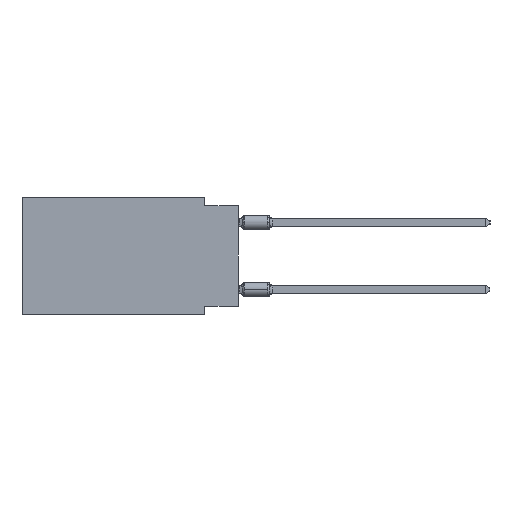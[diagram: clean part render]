
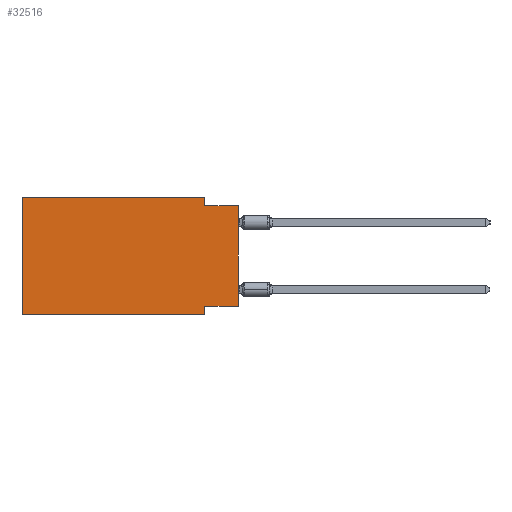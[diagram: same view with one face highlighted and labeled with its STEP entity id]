
A CAD part, left-side view. The second image highlights one B-rep face of the part: STEP entity #32516.
In plain terms, the highlighted planar face has unit normal (-1, 0, 0).
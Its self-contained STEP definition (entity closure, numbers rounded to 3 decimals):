
#209 = LINE ( 'NONE', #14138, #35410 ) ;
#517 = EDGE_CURVE ( 'NONE', #12664, #16205, #19904, .T. ) ;
#721 = EDGE_CURVE ( 'NONE', #12664, #32667, #12485, .T. ) ;
#1262 = CARTESIAN_POINT ( 'NONE',  ( 0., 2.54, -8.255 ) ) ;
#1575 = CARTESIAN_POINT ( 'NONE',  ( 0., 2.54, 0. ) ) ;
#2400 = CARTESIAN_POINT ( 'NONE',  ( 0., 16.383, 0. ) ) ;
#2664 = EDGE_CURVE ( 'NONE', #16205, #27501, #15067, .T. ) ;
#3215 = CARTESIAN_POINT ( 'NONE',  ( 0., 0., -0.635 ) ) ;
#3784 = CARTESIAN_POINT ( 'NONE',  ( 0., 0., -0.635 ) ) ;
#4337 = CARTESIAN_POINT ( 'NONE',  ( 0., 16.383, 0. ) ) ;
#5484 = VECTOR ( 'NONE', #33644, 1000. ) ;
#5692 = ORIENTED_EDGE ( 'NONE', *, *, #2664, .F. ) ;
#7178 = EDGE_CURVE ( 'NONE', #9628, #32667, #209, .T. ) ;
#7376 = DIRECTION ( 'NONE',  ( 1., 0., 0. ) ) ;
#7545 = CARTESIAN_POINT ( 'NONE',  ( 0., 0., -8.255 ) ) ;
#7728 = LINE ( 'NONE', #7545, #30053 ) ;
#8511 = EDGE_CURVE ( 'NONE', #9270, #9628, #7728, .T. ) ;
#8797 = EDGE_LOOP ( 'NONE', ( #23544, #12528, #15538, #5692, #13377, #13708, #22822, #29131 ) ) ;
#9270 = VERTEX_POINT ( 'NONE', #23692 ) ;
#9628 = VERTEX_POINT ( 'NONE', #1262 ) ;
#12485 = LINE ( 'NONE', #23487, #26822 ) ;
#12528 = ORIENTED_EDGE ( 'NONE', *, *, #15798, .F. ) ;
#12664 = VERTEX_POINT ( 'NONE', #22664 ) ;
#13008 = CARTESIAN_POINT ( 'NONE',  ( 0., 2.54, -8.89 ) ) ;
#13377 = ORIENTED_EDGE ( 'NONE', *, *, #517, .F. ) ;
#13708 = ORIENTED_EDGE ( 'NONE', *, *, #721, .T. ) ;
#14138 = CARTESIAN_POINT ( 'NONE',  ( 0., 2.54, -8.89 ) ) ;
#14813 = DIRECTION ( 'NONE',  ( 0., -1., 0. ) ) ;
#15067 = LINE ( 'NONE', #17786, #34929 ) ;
#15255 = VERTEX_POINT ( 'NONE', #3215 ) ;
#15538 = ORIENTED_EDGE ( 'NONE', *, *, #33761, .F. ) ;
#15556 = AXIS2_PLACEMENT_3D ( 'NONE', #4337, #7376, #29278 ) ;
#15798 = EDGE_CURVE ( 'NONE', #17107, #15255, #28551, .T. ) ;
#16205 = VERTEX_POINT ( 'NONE', #2400 ) ;
#16705 = VECTOR ( 'NONE', #28241, 1000. ) ;
#17107 = VERTEX_POINT ( 'NONE', #18580 ) ;
#17786 = CARTESIAN_POINT ( 'NONE',  ( 0., 16.383, 0. ) ) ;
#18580 = CARTESIAN_POINT ( 'NONE',  ( 0., 2.54, -0.635 ) ) ;
#19381 = DIRECTION ( 'NONE',  ( 0., 0., -1. ) ) ;
#19904 = LINE ( 'NONE', #22599, #5484 ) ;
#20783 = DIRECTION ( 'NONE',  ( 0., -1., 0. ) ) ;
#20915 = DIRECTION ( 'NONE',  ( 0., 0., -1. ) ) ;
#21738 = EDGE_CURVE ( 'NONE', #9270, #15255, #31151, .T. ) ;
#22599 = CARTESIAN_POINT ( 'NONE',  ( 0., 16.383, 0. ) ) ;
#22664 = CARTESIAN_POINT ( 'NONE',  ( 0., 16.383, -8.89 ) ) ;
#22822 = ORIENTED_EDGE ( 'NONE', *, *, #7178, .F. ) ;
#22825 = CARTESIAN_POINT ( 'NONE',  ( 0., 0., 0. ) ) ;
#23478 = FACE_OUTER_BOUND ( 'NONE', #8797, .T. ) ;
#23487 = CARTESIAN_POINT ( 'NONE',  ( 0., 16.383, -8.89 ) ) ;
#23544 = ORIENTED_EDGE ( 'NONE', *, *, #21738, .T. ) ;
#23692 = CARTESIAN_POINT ( 'NONE',  ( 0., 0., -8.255 ) ) ;
#23720 = DIRECTION ( 'NONE',  ( 0., -1., 0. ) ) ;
#26822 = VECTOR ( 'NONE', #20783, 1000. ) ;
#27069 = DIRECTION ( 'NONE',  ( 0., 1., 0. ) ) ;
#27501 = VERTEX_POINT ( 'NONE', #30721 ) ;
#28241 = DIRECTION ( 'NONE',  ( 0., 0., 1. ) ) ;
#28551 = LINE ( 'NONE', #3784, #35013 ) ;
#28903 = VECTOR ( 'NONE', #20915, 1000. ) ;
#29110 = PLANE ( 'NONE',  #15556 ) ;
#29131 = ORIENTED_EDGE ( 'NONE', *, *, #8511, .F. ) ;
#29278 = DIRECTION ( 'NONE',  ( 0., 0., -1. ) ) ;
#30053 = VECTOR ( 'NONE', #27069, 1000. ) ;
#30721 = CARTESIAN_POINT ( 'NONE',  ( 0., 2.54, 0. ) ) ;
#31151 = LINE ( 'NONE', #22825, #16705 ) ;
#31954 = LINE ( 'NONE', #1575, #28903 ) ;
#32516 = ADVANCED_FACE ( 'NONE', ( #23478 ), #29110, .F. ) ;
#32667 = VERTEX_POINT ( 'NONE', #13008 ) ;
#33644 = DIRECTION ( 'NONE',  ( 0., 0., 1. ) ) ;
#33761 = EDGE_CURVE ( 'NONE', #27501, #17107, #31954, .T. ) ;
#34929 = VECTOR ( 'NONE', #23720, 1000. ) ;
#35013 = VECTOR ( 'NONE', #14813, 1000. ) ;
#35410 = VECTOR ( 'NONE', #19381, 1000. ) ;
